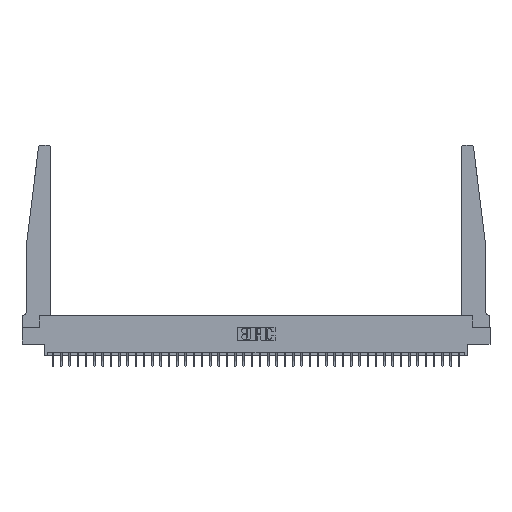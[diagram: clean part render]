
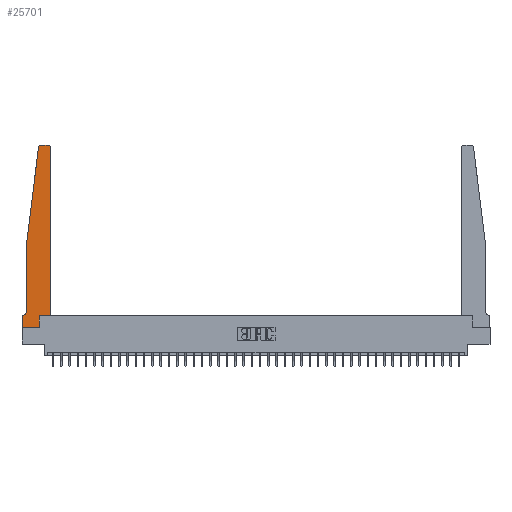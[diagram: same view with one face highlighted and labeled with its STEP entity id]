
A CAD part, top view. The second image highlights one B-rep face of the part: STEP entity #25701.
In plain terms, the highlighted planar face has unit normal (0, 0, 1).
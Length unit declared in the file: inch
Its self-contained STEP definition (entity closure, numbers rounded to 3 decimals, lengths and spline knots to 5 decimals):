
#13 = ORIENTED_EDGE ( 'NONE', *, *, #6015, .T. ) ;
#481 = VERTEX_POINT ( 'NONE', #14464 ) ;
#914 = ORIENTED_EDGE ( 'NONE', *, *, #1660, .T. ) ;
#1660 = EDGE_CURVE ( 'NONE', #36634, #11439, #22829, .T. ) ;
#1710 = LINE ( 'NONE', #8676, #9332 ) ;
#2700 = CIRCLE ( 'NONE', #8666, 0.03 ) ;
#3107 = VECTOR ( 'NONE', #30968, 39.37008 ) ;
#3116 = EDGE_CURVE ( 'NONE', #20268, #31461, #2700, .T. ) ;
#3846 = VERTEX_POINT ( 'NONE', #13529 ) ;
#3991 = VERTEX_POINT ( 'NONE', #14032 ) ;
#4070 = EDGE_CURVE ( 'NONE', #31476, #36634, #1710, .T. ) ;
#4871 = DIRECTION ( 'NONE',  ( 0., 1., 0. ) ) ;
#5354 = CARTESIAN_POINT ( 'NONE',  ( 0.425, 0.18, 0.37 ) ) ;
#5667 = CARTESIAN_POINT ( 'NONE',  ( 0.425, 0.18, 0.37 ) ) ;
#5722 = LINE ( 'NONE', #35684, #36176 ) ;
#5869 = CARTESIAN_POINT ( 'NONE',  ( 0., 0.1875, 0.37 ) ) ;
#6015 = EDGE_CURVE ( 'NONE', #14554, #3991, #14280, .T. ) ;
#7045 = FACE_OUTER_BOUND ( 'NONE', #26730, .T. ) ;
#7049 = VECTOR ( 'NONE', #30888, 39.37008 ) ;
#7150 = CARTESIAN_POINT ( 'NONE',  ( 0.395, 2.72, 0.37 ) ) ;
#7476 = EDGE_CURVE ( 'NONE', #3991, #481, #29185, .T. ) ;
#7719 = CARTESIAN_POINT ( 'NONE',  ( 0.27653, 2.75, 0.37 ) ) ;
#8312 = CARTESIAN_POINT ( 'NONE',  ( 0.065, 1.25, 0.37 ) ) ;
#8587 = CARTESIAN_POINT ( 'NONE',  ( 0.065, 1.25, 0.37 ) ) ;
#8666 = AXIS2_PLACEMENT_3D ( 'NONE', #9043, #28863, #11891 ) ;
#8676 = CARTESIAN_POINT ( 'NONE',  ( 0., 0., 0.37 ) ) ;
#9043 = CARTESIAN_POINT ( 'NONE',  ( 0.27653, 2.72, 0.37 ) ) ;
#9134 = CARTESIAN_POINT ( 'NONE',  ( 0.015, 0.2375, 0.37 ) ) ;
#9222 = PLANE ( 'NONE',  #19857 ) ;
#9332 = VECTOR ( 'NONE', #31315, 39.37008 ) ;
#9669 = AXIS2_PLACEMENT_3D ( 'NONE', #7150, #26997, #10009 ) ;
#10009 = DIRECTION ( 'NONE',  ( 1., 0., 0. ) ) ;
#10623 = VERTEX_POINT ( 'NONE', #14321 ) ;
#11439 = VERTEX_POINT ( 'NONE', #12107 ) ;
#11891 = DIRECTION ( 'NONE',  ( 1., 0., 0. ) ) ;
#11981 = DIRECTION ( 'NONE',  ( -1., 0., 0. ) ) ;
#12066 = DIRECTION ( 'NONE',  ( 0., 0., 1. ) ) ;
#12107 = CARTESIAN_POINT ( 'NONE',  ( 0.2605, 0.18, 0.37 ) ) ;
#12921 = VERTEX_POINT ( 'NONE', #8587 ) ;
#13362 = CARTESIAN_POINT ( 'NONE',  ( 0.2605, 0.18, 0.37 ) ) ;
#13529 = CARTESIAN_POINT ( 'NONE',  ( 0.065, 0.2375, 0.37 ) ) ;
#14032 = CARTESIAN_POINT ( 'NONE',  ( 0.425, 2.72, 0.37 ) ) ;
#14280 = LINE ( 'NONE', #5667, #22692 ) ;
#14321 = CARTESIAN_POINT ( 'NONE',  ( 0.015, 0.1875, 0.37 ) ) ;
#14464 = CARTESIAN_POINT ( 'NONE',  ( 0.395, 2.75, 0.37 ) ) ;
#14554 = VERTEX_POINT ( 'NONE', #35140 ) ;
#14961 = CARTESIAN_POINT ( 'NONE',  ( 0.25, 2.75, 0.37 ) ) ;
#15171 = VECTOR ( 'NONE', #18981, 39.37008 ) ;
#15299 = VECTOR ( 'NONE', #4871, 39.37008 ) ;
#15707 = ORIENTED_EDGE ( 'NONE', *, *, #19640, .T. ) ;
#15791 = AXIS2_PLACEMENT_3D ( 'NONE', #9134, #28946, #11981 ) ;
#16069 = LINE ( 'NONE', #21368, #30187 ) ;
#17038 = EDGE_CURVE ( 'NONE', #31461, #12921, #24872, .T. ) ;
#17730 = CARTESIAN_POINT ( 'NONE',  ( 0., 0.1875, 0.37 ) ) ;
#18705 = EDGE_CURVE ( 'NONE', #11439, #14554, #29658, .T. ) ;
#18884 = DIRECTION ( 'NONE',  ( 0., -1., 0. ) ) ;
#18981 = DIRECTION ( 'NONE',  ( 0., -1., 0. ) ) ;
#19640 = EDGE_CURVE ( 'NONE', #32522, #31476, #5722, .T. ) ;
#19857 = AXIS2_PLACEMENT_3D ( 'NONE', #17730, #12066, #31857 ) ;
#20268 = VERTEX_POINT ( 'NONE', #7719 ) ;
#20559 = ORIENTED_EDGE ( 'NONE', *, *, #18705, .T. ) ;
#20564 = DIRECTION ( 'NONE',  ( -1., 0., 0. ) ) ;
#21368 = CARTESIAN_POINT ( 'NONE',  ( 0.065, 0.1875, 0.37 ) ) ;
#21970 = ORIENTED_EDGE ( 'NONE', *, *, #26922, .T. ) ;
#22019 = CIRCLE ( 'NONE', #15791, 0.05 ) ;
#22178 = ORIENTED_EDGE ( 'NONE', *, *, #25703, .T. ) ;
#22692 = VECTOR ( 'NONE', #33993, 39.37008 ) ;
#22829 = LINE ( 'NONE', #13362, #15299 ) ;
#23572 = LINE ( 'NONE', #32978, #15171 ) ;
#23817 = ORIENTED_EDGE ( 'NONE', *, *, #30434, .T. ) ;
#24140 = DIRECTION ( 'NONE',  ( -1., 0., 0. ) ) ;
#24479 = EDGE_CURVE ( 'NONE', #10623, #32522, #16069, .T. ) ;
#24872 = LINE ( 'NONE', #8312, #3107 ) ;
#25701 = ADVANCED_FACE ( 'NONE', ( #7045 ), #9222, .T. ) ;
#25703 = EDGE_CURVE ( 'NONE', #481, #20268, #29654, .T. ) ;
#26730 = EDGE_LOOP ( 'NONE', ( #22178, #36273, #36306, #23817, #21970, #33040, #15707, #35652, #914, #20559, #13, #27343 ) ) ;
#26922 = EDGE_CURVE ( 'NONE', #3846, #10623, #22019, .T. ) ;
#26997 = DIRECTION ( 'NONE',  ( 0., 0., 1. ) ) ;
#27343 = ORIENTED_EDGE ( 'NONE', *, *, #7476, .T. ) ;
#28757 = CARTESIAN_POINT ( 'NONE',  ( 0., 0., 0.37 ) ) ;
#28863 = DIRECTION ( 'NONE',  ( 0., 0., 1. ) ) ;
#28946 = DIRECTION ( 'NONE',  ( 0., 0., -1. ) ) ;
#29185 = CIRCLE ( 'NONE', #9669, 0.03 ) ;
#29654 = LINE ( 'NONE', #14961, #36226 ) ;
#29658 = LINE ( 'NONE', #5354, #7049 ) ;
#30187 = VECTOR ( 'NONE', #24140, 39.37008 ) ;
#30434 = EDGE_CURVE ( 'NONE', #12921, #3846, #23572, .T. ) ;
#30888 = DIRECTION ( 'NONE',  ( 1., 0., 0. ) ) ;
#30968 = DIRECTION ( 'NONE',  ( -0.122, -0.992, 0. ) ) ;
#31315 = DIRECTION ( 'NONE',  ( 1., 0., 0. ) ) ;
#31461 = VERTEX_POINT ( 'NONE', #34248 ) ;
#31476 = VERTEX_POINT ( 'NONE', #28757 ) ;
#31857 = DIRECTION ( 'NONE',  ( 1., 0., 0. ) ) ;
#32362 = CARTESIAN_POINT ( 'NONE',  ( 0.2605, 0., 0.37 ) ) ;
#32522 = VERTEX_POINT ( 'NONE', #5869 ) ;
#32978 = CARTESIAN_POINT ( 'NONE',  ( 0.065, 1.25, 0.37 ) ) ;
#33040 = ORIENTED_EDGE ( 'NONE', *, *, #24479, .T. ) ;
#33993 = DIRECTION ( 'NONE',  ( 0., 1., 0. ) ) ;
#34248 = CARTESIAN_POINT ( 'NONE',  ( 0.24675, 2.72367, 0.37 ) ) ;
#35140 = CARTESIAN_POINT ( 'NONE',  ( 0.425, 0.18, 0.37 ) ) ;
#35652 = ORIENTED_EDGE ( 'NONE', *, *, #4070, .T. ) ;
#35684 = CARTESIAN_POINT ( 'NONE',  ( 0., 0., 0.37 ) ) ;
#36176 = VECTOR ( 'NONE', #18884, 39.37008 ) ;
#36226 = VECTOR ( 'NONE', #20564, 39.37008 ) ;
#36273 = ORIENTED_EDGE ( 'NONE', *, *, #3116, .T. ) ;
#36306 = ORIENTED_EDGE ( 'NONE', *, *, #17038, .T. ) ;
#36634 = VERTEX_POINT ( 'NONE', #32362 ) ;
